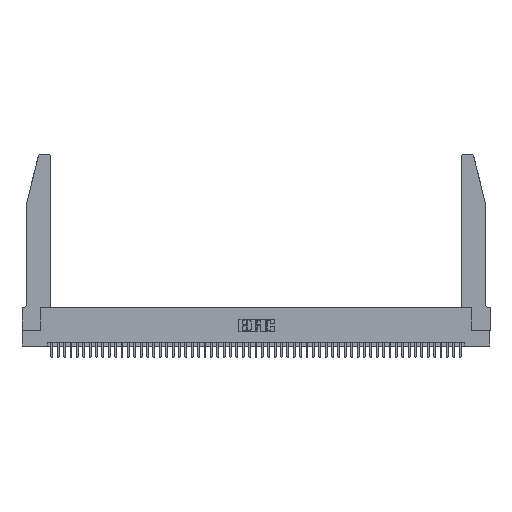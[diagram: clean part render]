
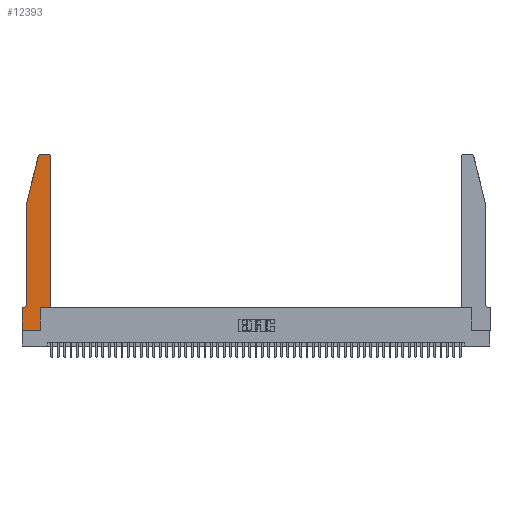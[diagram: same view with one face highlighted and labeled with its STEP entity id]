
A CAD part, top view. The second image highlights one B-rep face of the part: STEP entity #12393.
In plain terms, the highlighted planar face has unit normal (0, 0, 1).
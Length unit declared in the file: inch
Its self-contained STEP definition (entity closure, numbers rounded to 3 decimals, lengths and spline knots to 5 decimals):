
#13 = CARTESIAN_POINT ( 'NONE',  ( 0.0055, 0.35, 0.37 ) ) ;
#2313 = LINE ( 'NONE', #45008, #14682 ) ;
#2707 = DIRECTION ( 'NONE',  ( 0., 0., 1. ) ) ;
#2822 = VERTEX_POINT ( 'NONE', #21110 ) ;
#2860 = ORIENTED_EDGE ( 'NONE', *, *, #38982, .T. ) ;
#3273 = VERTEX_POINT ( 'NONE', #13 ) ;
#4071 = VERTEX_POINT ( 'NONE', #29643 ) ;
#4587 = DIRECTION ( 'NONE',  ( 0., 1., 0. ) ) ;
#4671 = ORIENTED_EDGE ( 'NONE', *, *, #22602, .T. ) ;
#4839 = LINE ( 'NONE', #46464, #45654 ) ;
#5893 = CARTESIAN_POINT ( 'NONE',  ( 0.0755, 0.42, 0.37 ) ) ;
#5939 = CARTESIAN_POINT ( 'NONE',  ( 0.0055, 0.42, 0.37 ) ) ;
#5956 = DIRECTION ( 'NONE',  ( 1., 0., 0. ) ) ;
#7170 = VECTOR ( 'NONE', #4587, 39.37008 ) ;
#7362 = VECTOR ( 'NONE', #13408, 39.37008 ) ;
#10109 = PLANE ( 'NONE',  #19720 ) ;
#10145 = DIRECTION ( 'NONE',  ( -1., 0., 0. ) ) ;
#10874 = VECTOR ( 'NONE', #23993, 39.37008 ) ;
#11182 = ORIENTED_EDGE ( 'NONE', *, *, #29420, .T. ) ;
#11331 = CARTESIAN_POINT ( 'NONE',  ( 0.2865, 0., 0.37 ) ) ;
#11546 = ORIENTED_EDGE ( 'NONE', *, *, #32252, .T. ) ;
#12037 = VERTEX_POINT ( 'NONE', #12280 ) ;
#12280 = CARTESIAN_POINT ( 'NONE',  ( 0.4505, 0.35, 0.37 ) ) ;
#12393 = ADVANCED_FACE ( 'NONE', ( #49480 ), #10109, .T. ) ;
#13311 = CARTESIAN_POINT ( 'NONE',  ( 0.25487, 2.72718, 0.37 ) ) ;
#13408 = DIRECTION ( 'NONE',  ( 1., 0., 0. ) ) ;
#13788 = LINE ( 'NONE', #26575, #34149 ) ;
#14130 = ORIENTED_EDGE ( 'NONE', *, *, #16787, .T. ) ;
#14247 = DIRECTION ( 'NONE',  ( 1., 0., 0. ) ) ;
#14682 = VECTOR ( 'NONE', #21025, 39.37008 ) ;
#15839 = EDGE_CURVE ( 'NONE', #30364, #41594, #18220, .T. ) ;
#16455 = ORIENTED_EDGE ( 'NONE', *, *, #15839, .T. ) ;
#16787 = EDGE_CURVE ( 'NONE', #43215, #3273, #51601, .T. ) ;
#17864 = AXIS2_PLACEMENT_3D ( 'NONE', #19760, #47979, #23836 ) ;
#18220 = LINE ( 'NONE', #49247, #7170 ) ;
#19398 = VERTEX_POINT ( 'NONE', #13311 ) ;
#19455 = ORIENTED_EDGE ( 'NONE', *, *, #25456, .T. ) ;
#19518 = EDGE_CURVE ( 'NONE', #49165, #40277, #4839, .T. ) ;
#19720 = AXIS2_PLACEMENT_3D ( 'NONE', #34515, #38559, #14247 ) ;
#19760 = CARTESIAN_POINT ( 'NONE',  ( 0.4205, 2.72, 0.37 ) ) ;
#20651 = DIRECTION ( 'NONE',  ( -0.239, -0.971, 0. ) ) ;
#20963 = EDGE_CURVE ( 'NONE', #41594, #12037, #38635, .T. ) ;
#21025 = DIRECTION ( 'NONE',  ( 0., -1., 0. ) ) ;
#21110 = CARTESIAN_POINT ( 'NONE',  ( 0., 0.35, 0.37 ) ) ;
#21752 = EDGE_CURVE ( 'NONE', #28816, #43215, #13788, .T. ) ;
#22310 = DIRECTION ( 'NONE',  ( -1., 0., 0. ) ) ;
#22602 = EDGE_CURVE ( 'NONE', #19398, #28816, #48550, .T. ) ;
#22834 = ORIENTED_EDGE ( 'NONE', *, *, #50324, .T. ) ;
#23541 = CARTESIAN_POINT ( 'NONE',  ( 0.2865, 0.35, 0.37 ) ) ;
#23836 = DIRECTION ( 'NONE',  ( 1., 0., 0. ) ) ;
#23993 = DIRECTION ( 'NONE',  ( 0., 1., 0. ) ) ;
#24566 = CARTESIAN_POINT ( 'NONE',  ( 0.0755, 2., 0.37 ) ) ;
#24950 = CARTESIAN_POINT ( 'NONE',  ( 0.4205, 2.75, 0.37 ) ) ;
#25456 = EDGE_CURVE ( 'NONE', #40277, #19398, #36936, .T. ) ;
#26575 = CARTESIAN_POINT ( 'NONE',  ( 0.0755, 2., 0.37 ) ) ;
#27155 = CARTESIAN_POINT ( 'NONE',  ( 0.0755, 0.35, 0.37 ) ) ;
#27407 = CARTESIAN_POINT ( 'NONE',  ( 0.284, 2.72, 0.37 ) ) ;
#27418 = ORIENTED_EDGE ( 'NONE', *, *, #21752, .T. ) ;
#27855 = ORIENTED_EDGE ( 'NONE', *, *, #20963, .T. ) ;
#28816 = VERTEX_POINT ( 'NONE', #34641 ) ;
#29029 = LINE ( 'NONE', #46566, #49178 ) ;
#29420 = EDGE_CURVE ( 'NONE', #48586, #30364, #29029, .T. ) ;
#29643 = CARTESIAN_POINT ( 'NONE',  ( 0.4505, 2.72, 0.37 ) ) ;
#30364 = VERTEX_POINT ( 'NONE', #11331 ) ;
#31440 = DIRECTION ( 'NONE',  ( 1., 0., 0. ) ) ;
#32252 = EDGE_CURVE ( 'NONE', #12037, #4071, #42047, .T. ) ;
#33617 = CARTESIAN_POINT ( 'NONE',  ( 0., 0., 0.37 ) ) ;
#34149 = VECTOR ( 'NONE', #46830, 39.37008 ) ;
#34515 = CARTESIAN_POINT ( 'NONE',  ( 0., 0.35, 0.37 ) ) ;
#34538 = ORIENTED_EDGE ( 'NONE', *, *, #19518, .T. ) ;
#34549 = DIRECTION ( 'NONE',  ( 0., 0., -1. ) ) ;
#34641 = CARTESIAN_POINT ( 'NONE',  ( 0.0755, 2., 0.37 ) ) ;
#36206 = EDGE_CURVE ( 'NONE', #3273, #2822, #44346, .T. ) ;
#36414 = EDGE_LOOP ( 'NONE', ( #34538, #19455, #4671, #27418, #14130, #37417, #22834, #11182, #16455, #27855, #11546, #2860 ) ) ;
#36936 = CIRCLE ( 'NONE', #41972, 0.03 ) ;
#37417 = ORIENTED_EDGE ( 'NONE', *, *, #36206, .T. ) ;
#38559 = DIRECTION ( 'NONE',  ( 0., 0., 1. ) ) ;
#38635 = LINE ( 'NONE', #49883, #7362 ) ;
#38982 = EDGE_CURVE ( 'NONE', #4071, #49165, #49144, .T. ) ;
#39106 = VECTOR ( 'NONE', #20651, 39.37008 ) ;
#40277 = VERTEX_POINT ( 'NONE', #48226 ) ;
#41594 = VERTEX_POINT ( 'NONE', #23541 ) ;
#41972 = AXIS2_PLACEMENT_3D ( 'NONE', #27407, #2707, #31440 ) ;
#42047 = LINE ( 'NONE', #48130, #10874 ) ;
#42758 = AXIS2_PLACEMENT_3D ( 'NONE', #5939, #34549, #10145 ) ;
#43215 = VERTEX_POINT ( 'NONE', #5893 ) ;
#44346 = LINE ( 'NONE', #27155, #51264 ) ;
#45008 = CARTESIAN_POINT ( 'NONE',  ( 0., 0., 0.37 ) ) ;
#45654 = VECTOR ( 'NONE', #22310, 39.37008 ) ;
#46464 = CARTESIAN_POINT ( 'NONE',  ( 0.2605, 2.75, 0.37 ) ) ;
#46566 = CARTESIAN_POINT ( 'NONE',  ( 0., 0., 0.37 ) ) ;
#46830 = DIRECTION ( 'NONE',  ( 0., -1., 0. ) ) ;
#47979 = DIRECTION ( 'NONE',  ( 0., 0., 1. ) ) ;
#48130 = CARTESIAN_POINT ( 'NONE',  ( 0.4505, 0.35, 0.37 ) ) ;
#48226 = CARTESIAN_POINT ( 'NONE',  ( 0.284, 2.75, 0.37 ) ) ;
#48550 = LINE ( 'NONE', #24566, #39106 ) ;
#48586 = VERTEX_POINT ( 'NONE', #33617 ) ;
#49144 = CIRCLE ( 'NONE', #17864, 0.03 ) ;
#49165 = VERTEX_POINT ( 'NONE', #24950 ) ;
#49178 = VECTOR ( 'NONE', #5956, 39.37008 ) ;
#49247 = CARTESIAN_POINT ( 'NONE',  ( 0.2865, 0.35, 0.37 ) ) ;
#49480 = FACE_OUTER_BOUND ( 'NONE', #36414, .T. ) ;
#49883 = CARTESIAN_POINT ( 'NONE',  ( 0.4505, 0.35, 0.37 ) ) ;
#50324 = EDGE_CURVE ( 'NONE', #2822, #48586, #2313, .T. ) ;
#51264 = VECTOR ( 'NONE', #51276, 39.37008 ) ;
#51276 = DIRECTION ( 'NONE',  ( -1., 0., 0. ) ) ;
#51601 = CIRCLE ( 'NONE', #42758, 0.07 ) ;
